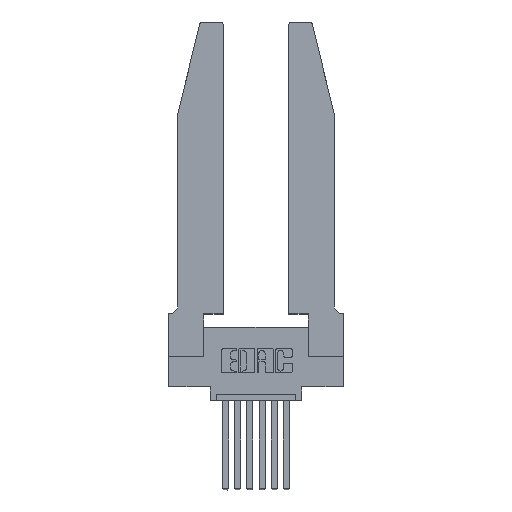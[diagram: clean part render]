
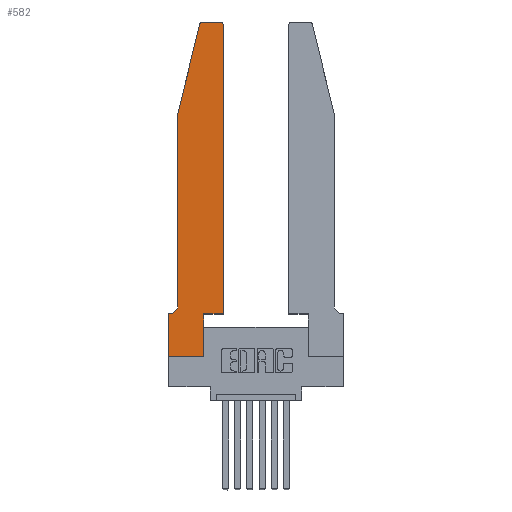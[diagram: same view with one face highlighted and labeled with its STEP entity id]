
A CAD part, top view. The second image highlights one B-rep face of the part: STEP entity #582.
In plain terms, the highlighted planar face has unit normal (0, 0, 1).
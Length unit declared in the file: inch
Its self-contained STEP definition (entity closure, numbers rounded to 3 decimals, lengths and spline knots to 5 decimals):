
#135 = CARTESIAN_POINT ( 'NONE',  ( 0.2865, 0.35, 0.37 ) ) ;
#508 = CARTESIAN_POINT ( 'NONE',  ( 0.4505, 0.35, 0.37 ) ) ;
#582 = ADVANCED_FACE ( 'NONE', ( #12732 ), #8122, .T. ) ;
#588 = DIRECTION ( 'NONE',  ( 1., 0., 0. ) ) ;
#602 = VECTOR ( 'NONE', #7664, 39.37008 ) ;
#791 = DIRECTION ( 'NONE',  ( -1., 0., 0. ) ) ;
#821 = CARTESIAN_POINT ( 'NONE',  ( 0.0755, 0.42, 0.37 ) ) ;
#951 = CARTESIAN_POINT ( 'NONE',  ( 0.284, 2.75, 0.37 ) ) ;
#1340 = DIRECTION ( 'NONE',  ( 1., 0., 0. ) ) ;
#1495 = ORIENTED_EDGE ( 'NONE', *, *, #11739, .T. ) ;
#1772 = DIRECTION ( 'NONE',  ( 0., -1., 0. ) ) ;
#1788 = EDGE_CURVE ( 'NONE', #6244, #9253, #9716, .T. ) ;
#2216 = VECTOR ( 'NONE', #6049, 39.37008 ) ;
#2422 = VERTEX_POINT ( 'NONE', #4293 ) ;
#2646 = CARTESIAN_POINT ( 'NONE',  ( 0.4205, 2.75, 0.37 ) ) ;
#2683 = DIRECTION ( 'NONE',  ( 0., 1., 0. ) ) ;
#2805 = CARTESIAN_POINT ( 'NONE',  ( 0., 0.35, 0.37 ) ) ;
#3011 = CARTESIAN_POINT ( 'NONE',  ( 0., 0., 0.37 ) ) ;
#3319 = VERTEX_POINT ( 'NONE', #4549 ) ;
#3342 = ORIENTED_EDGE ( 'NONE', *, *, #13195, .T. ) ;
#3521 = CARTESIAN_POINT ( 'NONE',  ( 0.0055, 0.35, 0.37 ) ) ;
#3559 = DIRECTION ( 'NONE',  ( -0.239, -0.971, 0. ) ) ;
#3588 = LINE ( 'NONE', #3011, #4787 ) ;
#3760 = CARTESIAN_POINT ( 'NONE',  ( 0.25487, 2.72718, 0.37 ) ) ;
#3774 = ORIENTED_EDGE ( 'NONE', *, *, #1788, .T. ) ;
#3878 = DIRECTION ( 'NONE',  ( 1., 0., 0. ) ) ;
#3912 = DIRECTION ( 'NONE',  ( 1., 0., 0. ) ) ;
#4080 = VERTEX_POINT ( 'NONE', #135 ) ;
#4258 = CARTESIAN_POINT ( 'NONE',  ( 0., 0., 0.37 ) ) ;
#4267 = ORIENTED_EDGE ( 'NONE', *, *, #9273, .T. ) ;
#4293 = CARTESIAN_POINT ( 'NONE',  ( 0., 0.35, 0.37 ) ) ;
#4455 = LINE ( 'NONE', #508, #13470 ) ;
#4549 = CARTESIAN_POINT ( 'NONE',  ( 0., 0., 0.37 ) ) ;
#4739 = EDGE_CURVE ( 'NONE', #2422, #3319, #9978, .T. ) ;
#4785 = ORIENTED_EDGE ( 'NONE', *, *, #11453, .T. ) ;
#4787 = VECTOR ( 'NONE', #13102, 39.37008 ) ;
#4837 = VERTEX_POINT ( 'NONE', #11529 ) ;
#4953 = VECTOR ( 'NONE', #7387, 39.37008 ) ;
#4959 = DIRECTION ( 'NONE',  ( 0., 0., 1. ) ) ;
#5121 = ORIENTED_EDGE ( 'NONE', *, *, #13351, .T. ) ;
#5455 = VECTOR ( 'NONE', #3559, 39.37008 ) ;
#5818 = VERTEX_POINT ( 'NONE', #951 ) ;
#5998 = VERTEX_POINT ( 'NONE', #3760 ) ;
#6049 = DIRECTION ( 'NONE',  ( 0., 1., 0. ) ) ;
#6227 = CARTESIAN_POINT ( 'NONE',  ( 0.0755, 2., 0.37 ) ) ;
#6244 = VERTEX_POINT ( 'NONE', #821 ) ;
#6523 = CIRCLE ( 'NONE', #8755, 0.03 ) ;
#6726 = VECTOR ( 'NONE', #1772, 39.37008 ) ;
#6734 = ORIENTED_EDGE ( 'NONE', *, *, #12773, .T. ) ;
#6864 = ORIENTED_EDGE ( 'NONE', *, *, #13654, .T. ) ;
#7149 = CIRCLE ( 'NONE', #12828, 0.03 ) ;
#7190 = CARTESIAN_POINT ( 'NONE',  ( 0.2865, 0.35, 0.37 ) ) ;
#7351 = EDGE_CURVE ( 'NONE', #11507, #4080, #11283, .T. ) ;
#7387 = DIRECTION ( 'NONE',  ( -1., 0., 0. ) ) ;
#7563 = LINE ( 'NONE', #11769, #4953 ) ;
#7664 = DIRECTION ( 'NONE',  ( 0., -1., 0. ) ) ;
#7825 = CARTESIAN_POINT ( 'NONE',  ( 0.0755, 2., 0.37 ) ) ;
#7873 = EDGE_CURVE ( 'NONE', #10144, #4837, #8747, .T. ) ;
#7899 = LINE ( 'NONE', #7825, #5455 ) ;
#7979 = CARTESIAN_POINT ( 'NONE',  ( 0.284, 2.72, 0.37 ) ) ;
#7992 = DIRECTION ( 'NONE',  ( -1., 0., 0. ) ) ;
#8122 = PLANE ( 'NONE',  #11656 ) ;
#8274 = AXIS2_PLACEMENT_3D ( 'NONE', #9717, #13869, #791 ) ;
#8747 = LINE ( 'NONE', #13662, #2216 ) ;
#8755 = AXIS2_PLACEMENT_3D ( 'NONE', #10406, #4959, #3912 ) ;
#9009 = CARTESIAN_POINT ( 'NONE',  ( 0.0755, 0.35, 0.37 ) ) ;
#9047 = DIRECTION ( 'NONE',  ( 0., 0., 1. ) ) ;
#9059 = CARTESIAN_POINT ( 'NONE',  ( 0.2865, 0., 0.37 ) ) ;
#9115 = EDGE_LOOP ( 'NONE', ( #5121, #4267, #6864, #1495, #3774, #4785, #13074, #11975, #13325, #6734, #13790, #3342 ) ) ;
#9253 = VERTEX_POINT ( 'NONE', #3521 ) ;
#9273 = EDGE_CURVE ( 'NONE', #5818, #5998, #7149, .T. ) ;
#9716 = CIRCLE ( 'NONE', #8274, 0.07 ) ;
#9717 = CARTESIAN_POINT ( 'NONE',  ( 0.0055, 0.42, 0.37 ) ) ;
#9927 = LINE ( 'NONE', #6227, #6726 ) ;
#9978 = LINE ( 'NONE', #4258, #602 ) ;
#10144 = VERTEX_POINT ( 'NONE', #13472 ) ;
#10406 = CARTESIAN_POINT ( 'NONE',  ( 0.4205, 2.72, 0.37 ) ) ;
#10778 = VECTOR ( 'NONE', #2683, 39.37008 ) ;
#11283 = LINE ( 'NONE', #7190, #10778 ) ;
#11289 = LINE ( 'NONE', #9009, #12665 ) ;
#11301 = CARTESIAN_POINT ( 'NONE',  ( 0.0755, 2., 0.37 ) ) ;
#11453 = EDGE_CURVE ( 'NONE', #9253, #2422, #11289, .T. ) ;
#11507 = VERTEX_POINT ( 'NONE', #9059 ) ;
#11529 = CARTESIAN_POINT ( 'NONE',  ( 0.4505, 2.72, 0.37 ) ) ;
#11656 = AXIS2_PLACEMENT_3D ( 'NONE', #2805, #12403, #588 ) ;
#11739 = EDGE_CURVE ( 'NONE', #13144, #6244, #9927, .T. ) ;
#11769 = CARTESIAN_POINT ( 'NONE',  ( 0.2605, 2.75, 0.37 ) ) ;
#11975 = ORIENTED_EDGE ( 'NONE', *, *, #12556, .T. ) ;
#12247 = VERTEX_POINT ( 'NONE', #2646 ) ;
#12403 = DIRECTION ( 'NONE',  ( 0., 0., 1. ) ) ;
#12556 = EDGE_CURVE ( 'NONE', #3319, #11507, #3588, .T. ) ;
#12665 = VECTOR ( 'NONE', #7992, 39.37008 ) ;
#12732 = FACE_OUTER_BOUND ( 'NONE', #9115, .T. ) ;
#12773 = EDGE_CURVE ( 'NONE', #4080, #10144, #4455, .T. ) ;
#12828 = AXIS2_PLACEMENT_3D ( 'NONE', #7979, #9047, #1340 ) ;
#13074 = ORIENTED_EDGE ( 'NONE', *, *, #4739, .T. ) ;
#13102 = DIRECTION ( 'NONE',  ( 1., 0., 0. ) ) ;
#13144 = VERTEX_POINT ( 'NONE', #11301 ) ;
#13195 = EDGE_CURVE ( 'NONE', #4837, #12247, #6523, .T. ) ;
#13325 = ORIENTED_EDGE ( 'NONE', *, *, #7351, .T. ) ;
#13351 = EDGE_CURVE ( 'NONE', #12247, #5818, #7563, .T. ) ;
#13470 = VECTOR ( 'NONE', #3878, 39.37008 ) ;
#13472 = CARTESIAN_POINT ( 'NONE',  ( 0.4505, 0.35, 0.37 ) ) ;
#13654 = EDGE_CURVE ( 'NONE', #5998, #13144, #7899, .T. ) ;
#13662 = CARTESIAN_POINT ( 'NONE',  ( 0.4505, 0.35, 0.37 ) ) ;
#13790 = ORIENTED_EDGE ( 'NONE', *, *, #7873, .T. ) ;
#13869 = DIRECTION ( 'NONE',  ( 0., 0., -1. ) ) ;
